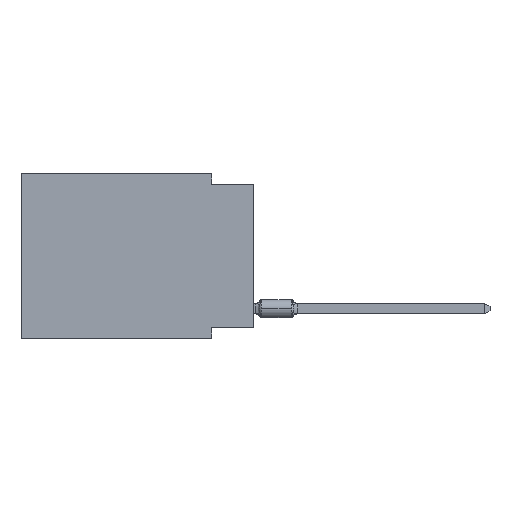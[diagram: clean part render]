
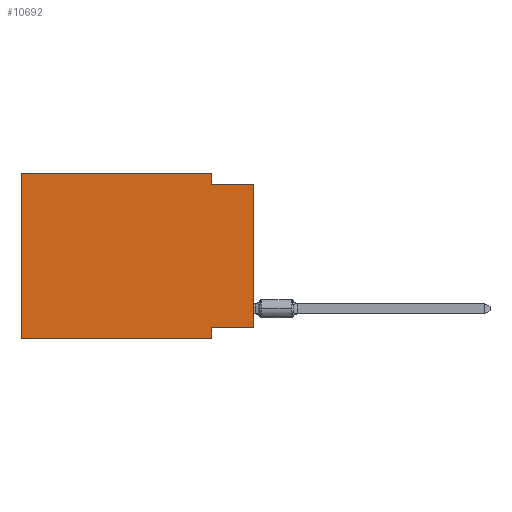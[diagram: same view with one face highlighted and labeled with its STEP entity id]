
A CAD part, left-side view. The second image highlights one B-rep face of the part: STEP entity #10692.
In plain terms, the highlighted planar face has unit normal (-1, 0, 0).
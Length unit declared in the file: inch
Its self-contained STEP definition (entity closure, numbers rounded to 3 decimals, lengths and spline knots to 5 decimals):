
#1625 = CARTESIAN_POINT ( 'NONE',  ( 0., 0.55, 0. ) ) ;
#1983 = DIRECTION ( 'NONE',  ( 0., 0., -1. ) ) ;
#2199 = DIRECTION ( 'NONE',  ( 1., 0., 0. ) ) ;
#3025 = CARTESIAN_POINT ( 'NONE',  ( 0., 0.1, -0.025 ) ) ;
#3202 = VECTOR ( 'NONE', #18488, 39.37008 ) ;
#4414 = LINE ( 'NONE', #15244, #3202 ) ;
#4748 = VERTEX_POINT ( 'NONE', #13309 ) ;
#5097 = LINE ( 'NONE', #1625, #36135 ) ;
#5668 = EDGE_CURVE ( 'NONE', #31283, #13142, #22883, .T. ) ;
#6208 = CARTESIAN_POINT ( 'NONE',  ( 0., 0., -0.025 ) ) ;
#6890 = CARTESIAN_POINT ( 'NONE',  ( 0., 0., 0. ) ) ;
#8863 = VERTEX_POINT ( 'NONE', #25801 ) ;
#9219 = EDGE_CURVE ( 'NONE', #39244, #34792, #24626, .T. ) ;
#9601 = LINE ( 'NONE', #38193, #15598 ) ;
#10692 = ADVANCED_FACE ( 'NONE', ( #23444 ), #41888, .F. ) ;
#12474 = DIRECTION ( 'NONE',  ( 0., 1., 0. ) ) ;
#13142 = VERTEX_POINT ( 'NONE', #40733 ) ;
#13155 = EDGE_CURVE ( 'NONE', #27855, #39244, #23665, .T. ) ;
#13309 = CARTESIAN_POINT ( 'NONE',  ( 0., 0.1, -0.39 ) ) ;
#13561 = ORIENTED_EDGE ( 'NONE', *, *, #43036, .F. ) ;
#13697 = DIRECTION ( 'NONE',  ( 0., -1., 0. ) ) ;
#13811 = LINE ( 'NONE', #6890, #39996 ) ;
#14235 = ORIENTED_EDGE ( 'NONE', *, *, #45158, .T. ) ;
#15236 = VECTOR ( 'NONE', #21632, 39.37008 ) ;
#15244 = CARTESIAN_POINT ( 'NONE',  ( 0., 0.55, 0. ) ) ;
#15598 = VECTOR ( 'NONE', #1983, 39.37008 ) ;
#15707 = CARTESIAN_POINT ( 'NONE',  ( 0., 0.55, 0. ) ) ;
#18051 = VECTOR ( 'NONE', #26882, 39.37008 ) ;
#18488 = DIRECTION ( 'NONE',  ( 0., 0., 1. ) ) ;
#21632 = DIRECTION ( 'NONE',  ( 0., -1., 0. ) ) ;
#22422 = DIRECTION ( 'NONE',  ( 0., -1., 0. ) ) ;
#22883 = LINE ( 'NONE', #26121, #43762 ) ;
#23312 = ORIENTED_EDGE ( 'NONE', *, *, #31900, .F. ) ;
#23444 = FACE_OUTER_BOUND ( 'NONE', #35874, .T. ) ;
#23665 = LINE ( 'NONE', #41650, #18051 ) ;
#24626 = LINE ( 'NONE', #38684, #15236 ) ;
#24845 = ORIENTED_EDGE ( 'NONE', *, *, #34867, .T. ) ;
#25419 = VERTEX_POINT ( 'NONE', #15707 ) ;
#25801 = CARTESIAN_POINT ( 'NONE',  ( 0., 0.55, -0.39 ) ) ;
#26121 = CARTESIAN_POINT ( 'NONE',  ( 0., 0., -0.365 ) ) ;
#26882 = DIRECTION ( 'NONE',  ( 0., 0., -1. ) ) ;
#26894 = CARTESIAN_POINT ( 'NONE',  ( 0., 0.55, 0. ) ) ;
#27066 = CARTESIAN_POINT ( 'NONE',  ( 0., 0.1, 0. ) ) ;
#27087 = LINE ( 'NONE', #34230, #33063 ) ;
#27855 = VERTEX_POINT ( 'NONE', #27066 ) ;
#27960 = ORIENTED_EDGE ( 'NONE', *, *, #13155, .F. ) ;
#28341 = DIRECTION ( 'NONE',  ( 0., 0., 1. ) ) ;
#29679 = ORIENTED_EDGE ( 'NONE', *, *, #9219, .F. ) ;
#31283 = VERTEX_POINT ( 'NONE', #33837 ) ;
#31900 = EDGE_CURVE ( 'NONE', #25419, #27855, #5097, .T. ) ;
#33063 = VECTOR ( 'NONE', #13697, 39.37008 ) ;
#33322 = AXIS2_PLACEMENT_3D ( 'NONE', #26894, #2199, #44664 ) ;
#33837 = CARTESIAN_POINT ( 'NONE',  ( 0., 0., -0.365 ) ) ;
#34230 = CARTESIAN_POINT ( 'NONE',  ( 0., 0.55, -0.39 ) ) ;
#34792 = VERTEX_POINT ( 'NONE', #6208 ) ;
#34867 = EDGE_CURVE ( 'NONE', #31283, #34792, #13811, .T. ) ;
#35814 = EDGE_CURVE ( 'NONE', #8863, #25419, #4414, .T. ) ;
#35874 = EDGE_LOOP ( 'NONE', ( #24845, #29679, #27960, #23312, #37776, #14235, #13561, #45618 ) ) ;
#36135 = VECTOR ( 'NONE', #22422, 39.37008 ) ;
#37776 = ORIENTED_EDGE ( 'NONE', *, *, #35814, .F. ) ;
#38193 = CARTESIAN_POINT ( 'NONE',  ( 0., 0.1, -0.39 ) ) ;
#38684 = CARTESIAN_POINT ( 'NONE',  ( 0., 0., -0.025 ) ) ;
#39244 = VERTEX_POINT ( 'NONE', #3025 ) ;
#39996 = VECTOR ( 'NONE', #28341, 39.37008 ) ;
#40733 = CARTESIAN_POINT ( 'NONE',  ( 0., 0.1, -0.365 ) ) ;
#41650 = CARTESIAN_POINT ( 'NONE',  ( 0., 0.1, 0. ) ) ;
#41888 = PLANE ( 'NONE',  #33322 ) ;
#43036 = EDGE_CURVE ( 'NONE', #13142, #4748, #9601, .T. ) ;
#43762 = VECTOR ( 'NONE', #12474, 39.37008 ) ;
#44664 = DIRECTION ( 'NONE',  ( 0., 0., -1. ) ) ;
#45158 = EDGE_CURVE ( 'NONE', #8863, #4748, #27087, .T. ) ;
#45618 = ORIENTED_EDGE ( 'NONE', *, *, #5668, .F. ) ;
